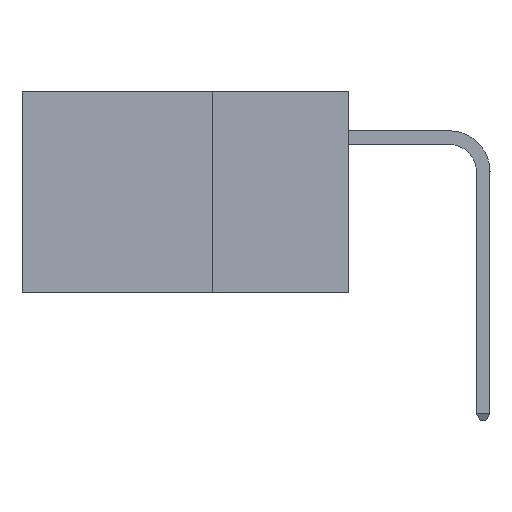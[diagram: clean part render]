
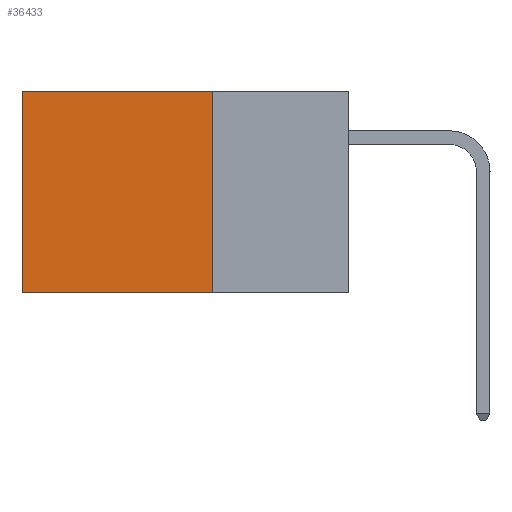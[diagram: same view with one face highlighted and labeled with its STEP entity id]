
A CAD part, left-side view. The second image highlights one B-rep face of the part: STEP entity #36433.
In plain terms, the highlighted planar face has unit normal (-1, 0, 0).
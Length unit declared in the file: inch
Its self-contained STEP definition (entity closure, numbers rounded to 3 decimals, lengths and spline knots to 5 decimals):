
#2657 = VECTOR ( 'NONE', #3183, 39.37008 ) ;
#3183 = DIRECTION ( 'NONE',  ( 0., 0., -1. ) ) ;
#3462 = LINE ( 'NONE', #24832, #7128 ) ;
#3606 = CARTESIAN_POINT ( 'NONE',  ( 0.2875, 0.25, 0. ) ) ;
#4053 = VECTOR ( 'NONE', #19763, 39.37008 ) ;
#7128 = VECTOR ( 'NONE', #27538, 39.37008 ) ;
#7954 = ORIENTED_EDGE ( 'NONE', *, *, #19761, .F. ) ;
#9170 = CARTESIAN_POINT ( 'NONE',  ( 0.2875, 0.25, 0. ) ) ;
#9417 = PLANE ( 'NONE',  #12536 ) ;
#10419 = EDGE_CURVE ( 'NONE', #24144, #18736, #25981, .T. ) ;
#10797 = LINE ( 'NONE', #9170, #24543 ) ;
#12536 = AXIS2_PLACEMENT_3D ( 'NONE', #18537, #24404, #27362 ) ;
#12908 = FACE_OUTER_BOUND ( 'NONE', #23494, .T. ) ;
#14734 = CARTESIAN_POINT ( 'NONE',  ( 0.2875, 0.25, -0.37 ) ) ;
#15675 = CARTESIAN_POINT ( 'NONE',  ( 0.2875, 0.25, 0. ) ) ;
#17302 = CARTESIAN_POINT ( 'NONE',  ( 0.2875, 0.6, 0. ) ) ;
#18537 = CARTESIAN_POINT ( 'NONE',  ( 0.2875, 0.25, 0. ) ) ;
#18736 = VERTEX_POINT ( 'NONE', #14734 ) ;
#19761 = EDGE_CURVE ( 'NONE', #18736, #31780, #3462, .T. ) ;
#19763 = DIRECTION ( 'NONE',  ( 0., 0., -1. ) ) ;
#21850 = ORIENTED_EDGE ( 'NONE', *, *, #24854, .T. ) ;
#22332 = CARTESIAN_POINT ( 'NONE',  ( 0.2875, 0.6, 0. ) ) ;
#23494 = EDGE_LOOP ( 'NONE', ( #25578, #7954, #37328, #21850 ) ) ;
#23809 = EDGE_CURVE ( 'NONE', #33871, #31780, #32386, .T. ) ;
#24140 = DIRECTION ( 'NONE',  ( 0., 1., 0. ) ) ;
#24144 = VERTEX_POINT ( 'NONE', #3606 ) ;
#24404 = DIRECTION ( 'NONE',  ( 1., 0., 0. ) ) ;
#24543 = VECTOR ( 'NONE', #24140, 39.37008 ) ;
#24832 = CARTESIAN_POINT ( 'NONE',  ( 0.2875, 0.25, -0.37 ) ) ;
#24854 = EDGE_CURVE ( 'NONE', #24144, #33871, #10797, .T. ) ;
#24875 = CARTESIAN_POINT ( 'NONE',  ( 0.2875, 0.6, -0.37 ) ) ;
#25578 = ORIENTED_EDGE ( 'NONE', *, *, #23809, .T. ) ;
#25981 = LINE ( 'NONE', #15675, #2657 ) ;
#27362 = DIRECTION ( 'NONE',  ( 0., 0., -1. ) ) ;
#27538 = DIRECTION ( 'NONE',  ( 0., 1., 0. ) ) ;
#31780 = VERTEX_POINT ( 'NONE', #24875 ) ;
#32386 = LINE ( 'NONE', #17302, #4053 ) ;
#33871 = VERTEX_POINT ( 'NONE', #22332 ) ;
#36433 = ADVANCED_FACE ( 'NONE', ( #12908 ), #9417, .F. ) ;
#37328 = ORIENTED_EDGE ( 'NONE', *, *, #10419, .F. ) ;
